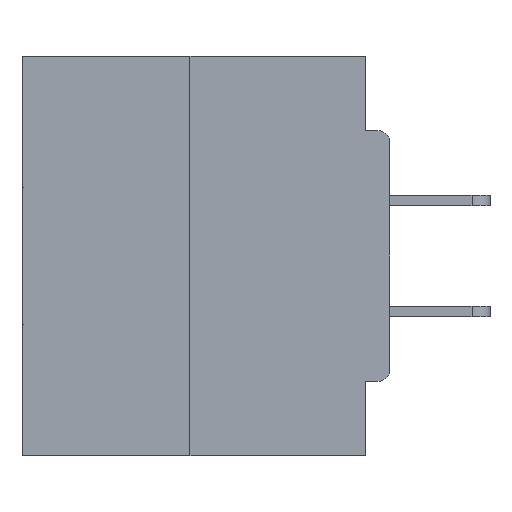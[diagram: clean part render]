
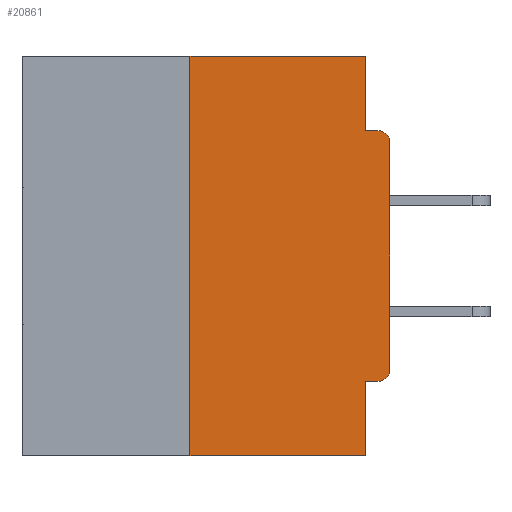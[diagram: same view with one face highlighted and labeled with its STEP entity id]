
A CAD part, left-side view. The second image highlights one B-rep face of the part: STEP entity #20861.
In plain terms, the highlighted planar face has unit normal (-1, 0, 0).
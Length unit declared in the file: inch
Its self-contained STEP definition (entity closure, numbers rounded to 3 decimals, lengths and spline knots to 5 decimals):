
#332 = ORIENTED_EDGE ( 'NONE', *, *, #14000, .F. ) ;
#633 = EDGE_CURVE ( 'NONE', #4290, #22357, #38080, .T. ) ;
#688 = CARTESIAN_POINT ( 'NONE',  ( 0., 0., -0.4065 ) ) ;
#1336 = CARTESIAN_POINT ( 'NONE',  ( 0., 0.25, -0.5 ) ) ;
#2371 = VECTOR ( 'NONE', #24743, 39.37008 ) ;
#2375 = VECTOR ( 'NONE', #2780, 39.37008 ) ;
#2780 = DIRECTION ( 'NONE',  ( 0., 0., 1. ) ) ;
#2816 = VECTOR ( 'NONE', #3232, 39.37008 ) ;
#3232 = DIRECTION ( 'NONE',  ( 0., -1., 0. ) ) ;
#3241 = DIRECTION ( 'NONE',  ( 0., -1., 0. ) ) ;
#3774 = ORIENTED_EDGE ( 'NONE', *, *, #34161, .F. ) ;
#4290 = VERTEX_POINT ( 'NONE', #16213 ) ;
#5877 = VERTEX_POINT ( 'NONE', #38699 ) ;
#6004 = EDGE_CURVE ( 'NONE', #28090, #4290, #28633, .T. ) ;
#6175 = VECTOR ( 'NONE', #3241, 39.37008 ) ;
#6606 = LINE ( 'NONE', #12567, #34940 ) ;
#6850 = DIRECTION ( 'NONE',  ( 0., 0., -1. ) ) ;
#6992 = AXIS2_PLACEMENT_3D ( 'NONE', #22315, #11160, #37513 ) ;
#7113 = CIRCLE ( 'NONE', #6992, 0.015 ) ;
#7235 = PLANE ( 'NONE',  #37514 ) ;
#8735 = CARTESIAN_POINT ( 'NONE',  ( 0., 0.46, 0. ) ) ;
#9269 = FACE_OUTER_BOUND ( 'NONE', #30009, .T. ) ;
#9720 = DIRECTION ( 'NONE',  ( 0., 0., 1. ) ) ;
#10092 = EDGE_CURVE ( 'NONE', #28090, #23182, #31175, .T. ) ;
#10100 = ORIENTED_EDGE ( 'NONE', *, *, #34499, .T. ) ;
#10276 = DIRECTION ( 'NONE',  ( 1., 0., 0. ) ) ;
#10496 = VERTEX_POINT ( 'NONE', #35539 ) ;
#11160 = DIRECTION ( 'NONE',  ( -1., 0., 0. ) ) ;
#11752 = EDGE_CURVE ( 'NONE', #10496, #5877, #20298, .T. ) ;
#12567 = CARTESIAN_POINT ( 'NONE',  ( 0., 0.031, -0.5 ) ) ;
#13377 = CARTESIAN_POINT ( 'NONE',  ( 0., 0., -0.3915 ) ) ;
#14000 = EDGE_CURVE ( 'NONE', #19546, #23182, #6606, .T. ) ;
#14202 = DIRECTION ( 'NONE',  ( 0., 0., -1. ) ) ;
#14707 = EDGE_CURVE ( 'NONE', #19245, #21698, #18402, .T. ) ;
#15278 = CARTESIAN_POINT ( 'NONE',  ( 0., 0.25, 0. ) ) ;
#15322 = CARTESIAN_POINT ( 'NONE',  ( 0., 0.031, 0. ) ) ;
#16033 = VECTOR ( 'NONE', #26274, 39.37008 ) ;
#16213 = CARTESIAN_POINT ( 'NONE',  ( 0., 0.25, 0. ) ) ;
#17259 = CARTESIAN_POINT ( 'NONE',  ( 0., 0.015, -0.1085 ) ) ;
#18402 = LINE ( 'NONE', #27046, #2375 ) ;
#19245 = VERTEX_POINT ( 'NONE', #13377 ) ;
#19546 = VERTEX_POINT ( 'NONE', #21069 ) ;
#20298 = LINE ( 'NONE', #32045, #16033 ) ;
#20836 = CARTESIAN_POINT ( 'NONE',  ( 0., 0.031, -0.5 ) ) ;
#20861 = ADVANCED_FACE ( 'NONE', ( #9269 ), #7235, .F. ) ;
#21069 = CARTESIAN_POINT ( 'NONE',  ( 0., 0.031, -0.4065 ) ) ;
#21298 = ORIENTED_EDGE ( 'NONE', *, *, #30596, .T. ) ;
#21311 = CARTESIAN_POINT ( 'NONE',  ( 0., 0.46, -0.5 ) ) ;
#21354 = ORIENTED_EDGE ( 'NONE', *, *, #6004, .F. ) ;
#21684 = VECTOR ( 'NONE', #27212, 39.37008 ) ;
#21698 = VERTEX_POINT ( 'NONE', #31844 ) ;
#21966 = CARTESIAN_POINT ( 'NONE',  ( 0., 0.46, 0. ) ) ;
#22142 = CIRCLE ( 'NONE', #35854, 0.015 ) ;
#22315 = CARTESIAN_POINT ( 'NONE',  ( 0., 0.015, -0.3915 ) ) ;
#22357 = VERTEX_POINT ( 'NONE', #38373 ) ;
#23130 = LINE ( 'NONE', #688, #2371 ) ;
#23182 = VERTEX_POINT ( 'NONE', #20836 ) ;
#24667 = ORIENTED_EDGE ( 'NONE', *, *, #11752, .F. ) ;
#24743 = DIRECTION ( 'NONE',  ( 0., 1., 0. ) ) ;
#25119 = EDGE_CURVE ( 'NONE', #26147, #19546, #23130, .T. ) ;
#26147 = VERTEX_POINT ( 'NONE', #38193 ) ;
#26274 = DIRECTION ( 'NONE',  ( 0., -1., 0. ) ) ;
#27046 = CARTESIAN_POINT ( 'NONE',  ( 0., 0., 0. ) ) ;
#27212 = DIRECTION ( 'NONE',  ( 0., 0., -1. ) ) ;
#28090 = VERTEX_POINT ( 'NONE', #1336 ) ;
#28633 = LINE ( 'NONE', #15278, #36175 ) ;
#30009 = EDGE_LOOP ( 'NONE', ( #32791, #21354, #38631, #332, #31557, #21298, #38978, #10100, #24667, #3774 ) ) ;
#30596 = EDGE_CURVE ( 'NONE', #26147, #19245, #7113, .T. ) ;
#30895 = DIRECTION ( 'NONE',  ( 0., 0., -1. ) ) ;
#31175 = LINE ( 'NONE', #21311, #6175 ) ;
#31557 = ORIENTED_EDGE ( 'NONE', *, *, #25119, .F. ) ;
#31844 = CARTESIAN_POINT ( 'NONE',  ( 0., 0., -0.1085 ) ) ;
#32045 = CARTESIAN_POINT ( 'NONE',  ( 0., 0., -0.0935 ) ) ;
#32791 = ORIENTED_EDGE ( 'NONE', *, *, #633, .F. ) ;
#34161 = EDGE_CURVE ( 'NONE', #22357, #10496, #37633, .T. ) ;
#34499 = EDGE_CURVE ( 'NONE', #21698, #5877, #22142, .T. ) ;
#34940 = VECTOR ( 'NONE', #30895, 39.37008 ) ;
#35539 = CARTESIAN_POINT ( 'NONE',  ( 0., 0.031, -0.0935 ) ) ;
#35854 = AXIS2_PLACEMENT_3D ( 'NONE', #17259, #38167, #14202 ) ;
#36175 = VECTOR ( 'NONE', #9720, 39.37008 ) ;
#37513 = DIRECTION ( 'NONE',  ( 0., 0., -1. ) ) ;
#37514 = AXIS2_PLACEMENT_3D ( 'NONE', #21966, #10276, #6850 ) ;
#37633 = LINE ( 'NONE', #15322, #21684 ) ;
#38080 = LINE ( 'NONE', #8735, #2816 ) ;
#38167 = DIRECTION ( 'NONE',  ( -1., 0., 0. ) ) ;
#38193 = CARTESIAN_POINT ( 'NONE',  ( 0., 0.015, -0.4065 ) ) ;
#38373 = CARTESIAN_POINT ( 'NONE',  ( 0., 0.031, 0. ) ) ;
#38631 = ORIENTED_EDGE ( 'NONE', *, *, #10092, .T. ) ;
#38699 = CARTESIAN_POINT ( 'NONE',  ( 0., 0.015, -0.0935 ) ) ;
#38978 = ORIENTED_EDGE ( 'NONE', *, *, #14707, .T. ) ;
